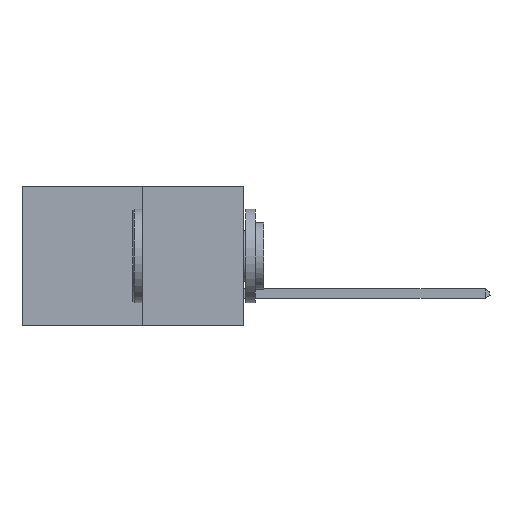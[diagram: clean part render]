
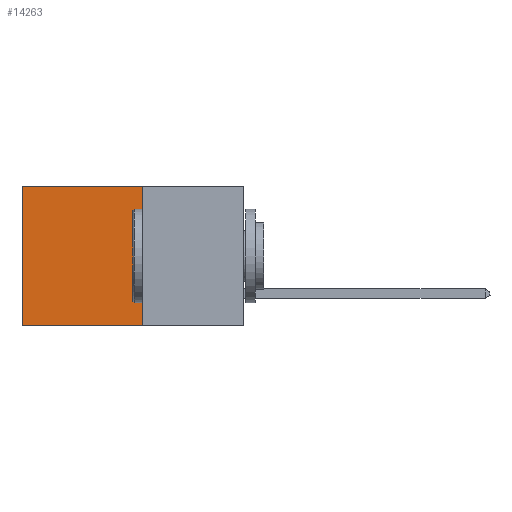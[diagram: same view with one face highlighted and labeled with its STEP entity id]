
A CAD part, left-side view. The second image highlights one B-rep face of the part: STEP entity #14263.
In plain terms, the highlighted planar face has unit normal (-1, 0, 0).
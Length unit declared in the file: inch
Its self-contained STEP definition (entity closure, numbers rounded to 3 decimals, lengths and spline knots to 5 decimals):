
#545 = DIRECTION ( 'NONE',  ( 0., 1., 0. ) ) ;
#971 = DIRECTION ( 'NONE',  ( 1., 0., 0. ) ) ;
#1590 = EDGE_CURVE ( 'NONE', #17275, #5347, #5129, .T. ) ;
#1727 = EDGE_LOOP ( 'NONE', ( #17789, #14807, #5536, #8061 ) ) ;
#2274 = LINE ( 'NONE', #13804, #16667 ) ;
#2382 = CARTESIAN_POINT ( 'NONE',  ( 0.277, 0.27, -0.37 ) ) ;
#3326 = CARTESIAN_POINT ( 'NONE',  ( 0.277, 0.27, 0. ) ) ;
#4116 = CARTESIAN_POINT ( 'NONE',  ( 0.277, 0.27, -0.37 ) ) ;
#5125 = CARTESIAN_POINT ( 'NONE',  ( 0.277, 0.27, -0.37 ) ) ;
#5129 = LINE ( 'NONE', #4116, #12099 ) ;
#5347 = VERTEX_POINT ( 'NONE', #17477 ) ;
#5403 = AXIS2_PLACEMENT_3D ( 'NONE', #7906, #971, #10683 ) ;
#5536 = ORIENTED_EDGE ( 'NONE', *, *, #15598, .F. ) ;
#5877 = EDGE_CURVE ( 'NONE', #5987, #16358, #10881, .T. ) ;
#5987 = VERTEX_POINT ( 'NONE', #11917 ) ;
#6530 = DIRECTION ( 'NONE',  ( 0., 0., -1. ) ) ;
#7906 = CARTESIAN_POINT ( 'NONE',  ( 0.277, 0.27, -0.37 ) ) ;
#8061 = ORIENTED_EDGE ( 'NONE', *, *, #5877, .T. ) ;
#9923 = FACE_OUTER_BOUND ( 'NONE', #1727, .T. ) ;
#10007 = EDGE_CURVE ( 'NONE', #16358, #5347, #2274, .T. ) ;
#10683 = DIRECTION ( 'NONE',  ( 0., 0., -1. ) ) ;
#10881 = LINE ( 'NONE', #3326, #12868 ) ;
#11917 = CARTESIAN_POINT ( 'NONE',  ( 0.277, 0.27, 0. ) ) ;
#12099 = VECTOR ( 'NONE', #13882, 39.37008 ) ;
#12868 = VECTOR ( 'NONE', #545, 39.37008 ) ;
#13165 = VECTOR ( 'NONE', #6530, 39.37008 ) ;
#13591 = LINE ( 'NONE', #5125, #13165 ) ;
#13804 = CARTESIAN_POINT ( 'NONE',  ( 0.277, 0.59, -0.37 ) ) ;
#13882 = DIRECTION ( 'NONE',  ( 0., 1., 0. ) ) ;
#14263 = ADVANCED_FACE ( 'NONE', ( #9923 ), #17649, .F. ) ;
#14807 = ORIENTED_EDGE ( 'NONE', *, *, #1590, .F. ) ;
#15598 = EDGE_CURVE ( 'NONE', #5987, #17275, #13591, .T. ) ;
#15768 = CARTESIAN_POINT ( 'NONE',  ( 0.277, 0.59, 0. ) ) ;
#16358 = VERTEX_POINT ( 'NONE', #15768 ) ;
#16667 = VECTOR ( 'NONE', #17999, 39.37008 ) ;
#17275 = VERTEX_POINT ( 'NONE', #2382 ) ;
#17477 = CARTESIAN_POINT ( 'NONE',  ( 0.277, 0.59, -0.37 ) ) ;
#17649 = PLANE ( 'NONE',  #5403 ) ;
#17789 = ORIENTED_EDGE ( 'NONE', *, *, #10007, .T. ) ;
#17999 = DIRECTION ( 'NONE',  ( 0., 0., -1. ) ) ;
